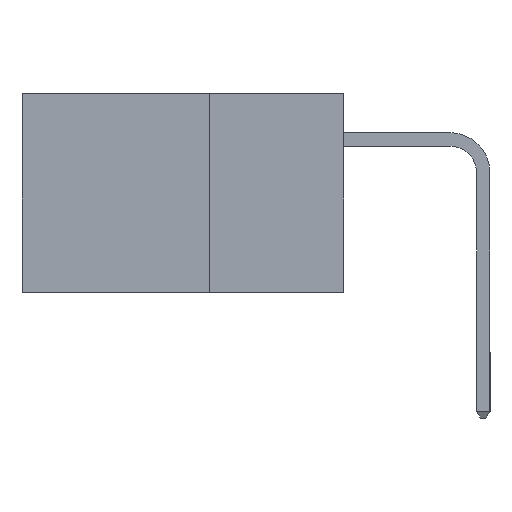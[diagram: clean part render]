
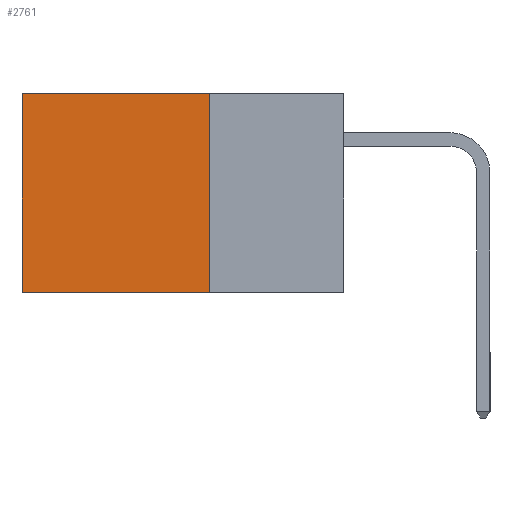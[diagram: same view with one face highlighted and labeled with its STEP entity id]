
A CAD part, left-side view. The second image highlights one B-rep face of the part: STEP entity #2761.
In plain terms, the highlighted planar face has unit normal (-1, 0, 0).
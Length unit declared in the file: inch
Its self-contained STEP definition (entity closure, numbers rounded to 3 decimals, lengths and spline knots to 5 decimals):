
#8 = EDGE_CURVE ( 'NONE', #10068, #3792, #3874, .T. ) ;
#141 = DIRECTION ( 'NONE',  ( 0., 0., -1. ) ) ;
#740 = DIRECTION ( 'NONE',  ( 0., 0., -1. ) ) ;
#814 = CARTESIAN_POINT ( 'NONE',  ( 0.298, 0.25, 0. ) ) ;
#1149 = CARTESIAN_POINT ( 'NONE',  ( 0.298, 0.6, 0. ) ) ;
#1176 = CARTESIAN_POINT ( 'NONE',  ( 0.298, 0.25, 0. ) ) ;
#1223 = DIRECTION ( 'NONE',  ( 0., 0., -1. ) ) ;
#1798 = CARTESIAN_POINT ( 'NONE',  ( 0.298, 0.6, -0.37 ) ) ;
#2150 = EDGE_LOOP ( 'NONE', ( #6191, #6187, #8584, #9068 ) ) ;
#2761 = ADVANCED_FACE ( 'NONE', ( #10563 ), #10011, .F. ) ;
#2781 = LINE ( 'NONE', #1176, #6783 ) ;
#3365 = VECTOR ( 'NONE', #9254, 39.37008 ) ;
#3792 = VERTEX_POINT ( 'NONE', #1149 ) ;
#3874 = LINE ( 'NONE', #8114, #12052 ) ;
#4157 = VECTOR ( 'NONE', #1223, 39.37008 ) ;
#4179 = CARTESIAN_POINT ( 'NONE',  ( 0.298, 0.6, 0. ) ) ;
#4509 = VERTEX_POINT ( 'NONE', #6678 ) ;
#5082 = DIRECTION ( 'NONE',  ( 0., 1., 0. ) ) ;
#5428 = DIRECTION ( 'NONE',  ( 1., 0., 0. ) ) ;
#5430 = EDGE_CURVE ( 'NONE', #3792, #8185, #10639, .T. ) ;
#6178 = LINE ( 'NONE', #12089, #3365 ) ;
#6187 = ORIENTED_EDGE ( 'NONE', *, *, #7600, .F. ) ;
#6191 = ORIENTED_EDGE ( 'NONE', *, *, #5430, .T. ) ;
#6380 = CARTESIAN_POINT ( 'NONE',  ( 0.298, 0.25, 0. ) ) ;
#6678 = CARTESIAN_POINT ( 'NONE',  ( 0.298, 0.25, -0.37 ) ) ;
#6783 = VECTOR ( 'NONE', #141, 39.37008 ) ;
#7600 = EDGE_CURVE ( 'NONE', #4509, #8185, #6178, .T. ) ;
#8114 = CARTESIAN_POINT ( 'NONE',  ( 0.298, 0.25, 0. ) ) ;
#8185 = VERTEX_POINT ( 'NONE', #1798 ) ;
#8584 = ORIENTED_EDGE ( 'NONE', *, *, #11798, .F. ) ;
#9068 = ORIENTED_EDGE ( 'NONE', *, *, #8, .T. ) ;
#9254 = DIRECTION ( 'NONE',  ( 0., 1., 0. ) ) ;
#10011 = PLANE ( 'NONE',  #11986 ) ;
#10068 = VERTEX_POINT ( 'NONE', #814 ) ;
#10563 = FACE_OUTER_BOUND ( 'NONE', #2150, .T. ) ;
#10639 = LINE ( 'NONE', #4179, #4157 ) ;
#11798 = EDGE_CURVE ( 'NONE', #10068, #4509, #2781, .T. ) ;
#11986 = AXIS2_PLACEMENT_3D ( 'NONE', #6380, #5428, #740 ) ;
#12052 = VECTOR ( 'NONE', #5082, 39.37008 ) ;
#12089 = CARTESIAN_POINT ( 'NONE',  ( 0.298, 0.25, -0.37 ) ) ;
